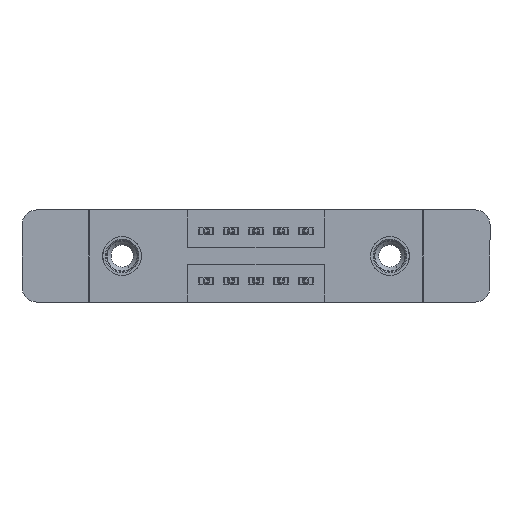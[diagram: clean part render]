
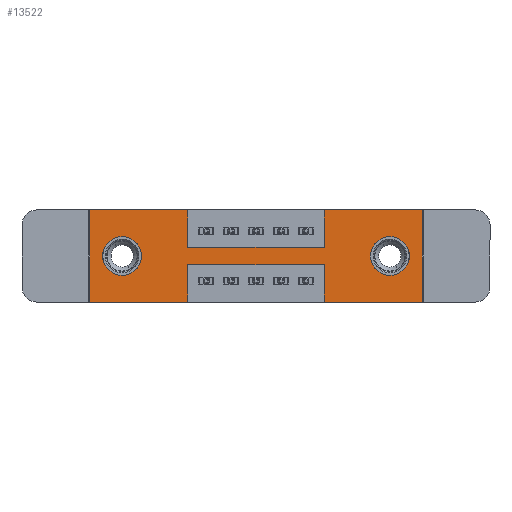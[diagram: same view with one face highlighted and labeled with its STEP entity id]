
A CAD part, front view. The second image highlights one B-rep face of the part: STEP entity #13522.
In plain terms, the highlighted planar face has unit normal (0, -1, 0).
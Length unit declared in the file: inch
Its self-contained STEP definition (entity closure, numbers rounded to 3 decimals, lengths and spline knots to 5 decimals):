
#14 = ORIENTED_EDGE ( 'NONE', *, *, #12716, .F. ) ;
#40 = CARTESIAN_POINT ( 'NONE',  ( 0.3925, 0., -0.15 ) ) ;
#54 = VERTEX_POINT ( 'NONE', #1777 ) ;
#109 = DIRECTION ( 'NONE',  ( 0., 0., 1. ) ) ;
#143 = CARTESIAN_POINT ( 'NONE',  ( 0.13, 0., -0.263 ) ) ;
#145 = CIRCLE ( 'NONE', #7231, 0.078 ) ;
#242 = CIRCLE ( 'NONE', #5730, 0.078 ) ;
#367 = DIRECTION ( 'NONE',  ( 0., 0., 1. ) ) ;
#396 = VERTEX_POINT ( 'NONE', #4580 ) ;
#408 = EDGE_CURVE ( 'NONE', #1911, #396, #1537, .T. ) ;
#434 = VECTOR ( 'NONE', #10616, 39.37008 ) ;
#489 = EDGE_CURVE ( 'NONE', #2141, #800, #8428, .T. ) ;
#511 = CARTESIAN_POINT ( 'NONE',  ( 0.9425, 0., 0. ) ) ;
#569 = DIRECTION ( 'NONE',  ( 0., 0., -1. ) ) ;
#647 = DIRECTION ( 'NONE',  ( -1., 0., 0. ) ) ;
#788 = CARTESIAN_POINT ( 'NONE',  ( 0.3925, 0., -0.37 ) ) ;
#800 = VERTEX_POINT ( 'NONE', #5962 ) ;
#908 = VERTEX_POINT ( 'NONE', #143 ) ;
#941 = ORIENTED_EDGE ( 'NONE', *, *, #489, .F. ) ;
#1104 = VERTEX_POINT ( 'NONE', #11388 ) ;
#1537 = CIRCLE ( 'NONE', #7495, 0.078 ) ;
#1569 = CARTESIAN_POINT ( 'NONE',  ( 0., 0., -0.37 ) ) ;
#1573 = CIRCLE ( 'NONE', #5460, 0.078 ) ;
#1625 = DIRECTION ( 'NONE',  ( 0., 1., 0. ) ) ;
#1772 = EDGE_CURVE ( 'NONE', #54, #3275, #6254, .T. ) ;
#1777 = CARTESIAN_POINT ( 'NONE',  ( 0.9425, 0., -0.22 ) ) ;
#1802 = CARTESIAN_POINT ( 'NONE',  ( 0.9425, 0., -0.37 ) ) ;
#1911 = VERTEX_POINT ( 'NONE', #5954 ) ;
#1930 = ORIENTED_EDGE ( 'NONE', *, *, #1772, .F. ) ;
#2028 = CARTESIAN_POINT ( 'NONE',  ( 0.9425, 0., -0.37 ) ) ;
#2094 = ORIENTED_EDGE ( 'NONE', *, *, #10803, .F. ) ;
#2141 = VERTEX_POINT ( 'NONE', #4910 ) ;
#2240 = CARTESIAN_POINT ( 'NONE',  ( 1.205, 0., -0.185 ) ) ;
#2312 = EDGE_CURVE ( 'NONE', #8408, #2580, #8908, .T. ) ;
#2437 = VERTEX_POINT ( 'NONE', #9054 ) ;
#2528 = VECTOR ( 'NONE', #7247, 39.37008 ) ;
#2580 = VERTEX_POINT ( 'NONE', #13516 ) ;
#2590 = DIRECTION ( 'NONE',  ( 0., -1., 0. ) ) ;
#2774 = CARTESIAN_POINT ( 'NONE',  ( 0., 0., -0.37 ) ) ;
#2799 = ORIENTED_EDGE ( 'NONE', *, *, #12905, .T. ) ;
#2869 = LINE ( 'NONE', #7093, #11901 ) ;
#2993 = DIRECTION ( 'NONE',  ( 0., 0., -1. ) ) ;
#3033 = EDGE_CURVE ( 'NONE', #3275, #1104, #11607, .T. ) ;
#3177 = LINE ( 'NONE', #13793, #10722 ) ;
#3210 = DIRECTION ( 'NONE',  ( 0., 0., 1. ) ) ;
#3251 = ORIENTED_EDGE ( 'NONE', *, *, #6600, .F. ) ;
#3275 = VERTEX_POINT ( 'NONE', #3446 ) ;
#3441 = CARTESIAN_POINT ( 'NONE',  ( 0.9425, 0., 0. ) ) ;
#3446 = CARTESIAN_POINT ( 'NONE',  ( 0.3925, 0., -0.22 ) ) ;
#3498 = DIRECTION ( 'NONE',  ( 0., 1., 0. ) ) ;
#3857 = VECTOR ( 'NONE', #13791, 39.37008 ) ;
#3929 = CARTESIAN_POINT ( 'NONE',  ( 1.335, 0., 0. ) ) ;
#3960 = ORIENTED_EDGE ( 'NONE', *, *, #13462, .F. ) ;
#4412 = DIRECTION ( 'NONE',  ( 1., 0., 0. ) ) ;
#4465 = DIRECTION ( 'NONE',  ( 0., 0., -1. ) ) ;
#4484 = DIRECTION ( 'NONE',  ( 0., 0., 1. ) ) ;
#4497 = VECTOR ( 'NONE', #4484, 39.37008 ) ;
#4580 = CARTESIAN_POINT ( 'NONE',  ( 1.205, 0., -0.263 ) ) ;
#4705 = VECTOR ( 'NONE', #2993, 39.37008 ) ;
#4761 = EDGE_LOOP ( 'NONE', ( #12959, #2799 ) ) ;
#4842 = ORIENTED_EDGE ( 'NONE', *, *, #13003, .F. ) ;
#4910 = CARTESIAN_POINT ( 'NONE',  ( 1.335, 0., 0. ) ) ;
#5101 = ORIENTED_EDGE ( 'NONE', *, *, #8015, .F. ) ;
#5460 = AXIS2_PLACEMENT_3D ( 'NONE', #2240, #13506, #4465 ) ;
#5730 = AXIS2_PLACEMENT_3D ( 'NONE', #5948, #12604, #109 ) ;
#5835 = ORIENTED_EDGE ( 'NONE', *, *, #12366, .F. ) ;
#5948 = CARTESIAN_POINT ( 'NONE',  ( 0.13, 0., -0.185 ) ) ;
#5954 = CARTESIAN_POINT ( 'NONE',  ( 1.205, 0., -0.107 ) ) ;
#5962 = CARTESIAN_POINT ( 'NONE',  ( 1.335, 0., -0.37 ) ) ;
#6108 = VECTOR ( 'NONE', #13656, 39.37008 ) ;
#6136 = LINE ( 'NONE', #11443, #4705 ) ;
#6254 = LINE ( 'NONE', #14079, #434 ) ;
#6389 = VECTOR ( 'NONE', #367, 39.37008 ) ;
#6572 = VERTEX_POINT ( 'NONE', #10578 ) ;
#6600 = EDGE_CURVE ( 'NONE', #2437, #8408, #6136, .T. ) ;
#7039 = VECTOR ( 'NONE', #7356, 39.37008 ) ;
#7068 = LINE ( 'NONE', #2774, #6108 ) ;
#7093 = CARTESIAN_POINT ( 'NONE',  ( 0., 0., -0.37 ) ) ;
#7224 = VERTEX_POINT ( 'NONE', #2028 ) ;
#7231 = AXIS2_PLACEMENT_3D ( 'NONE', #11948, #3498, #3210 ) ;
#7247 = DIRECTION ( 'NONE',  ( 0., 0., 1. ) ) ;
#7282 = CARTESIAN_POINT ( 'NONE',  ( 1.205, 0., -0.185 ) ) ;
#7356 = DIRECTION ( 'NONE',  ( 0., 0., -1. ) ) ;
#7495 = AXIS2_PLACEMENT_3D ( 'NONE', #7282, #1625, #11649 ) ;
#8015 = EDGE_CURVE ( 'NONE', #9460, #6572, #8506, .T. ) ;
#8163 = PLANE ( 'NONE',  #10294 ) ;
#8310 = EDGE_LOOP ( 'NONE', ( #13351, #1930, #4842, #3960, #941, #8535, #14, #8772, #3251, #5835, #5101, #2094 ) ) ;
#8333 = VERTEX_POINT ( 'NONE', #9343 ) ;
#8399 = CARTESIAN_POINT ( 'NONE',  ( 0., 0., 0. ) ) ;
#8408 = VERTEX_POINT ( 'NONE', #10776 ) ;
#8428 = LINE ( 'NONE', #3929, #7039 ) ;
#8506 = LINE ( 'NONE', #8836, #4497 ) ;
#8535 = ORIENTED_EDGE ( 'NONE', *, *, #11397, .F. ) ;
#8772 = ORIENTED_EDGE ( 'NONE', *, *, #2312, .F. ) ;
#8836 = CARTESIAN_POINT ( 'NONE',  ( 0., 0., 0. ) ) ;
#8908 = LINE ( 'NONE', #40, #12082 ) ;
#9054 = CARTESIAN_POINT ( 'NONE',  ( 0.3925, 0., 0. ) ) ;
#9343 = CARTESIAN_POINT ( 'NONE',  ( 0.13, 0., -0.107 ) ) ;
#9457 = EDGE_CURVE ( 'NONE', #8333, #908, #145, .T. ) ;
#9460 = VERTEX_POINT ( 'NONE', #13091 ) ;
#9608 = VECTOR ( 'NONE', #12965, 39.37008 ) ;
#9857 = EDGE_LOOP ( 'NONE', ( #10556, #12037 ) ) ;
#10169 = FACE_BOUND ( 'NONE', #4761, .T. ) ;
#10198 = VERTEX_POINT ( 'NONE', #3441 ) ;
#10243 = FACE_OUTER_BOUND ( 'NONE', #8310, .T. ) ;
#10294 = AXIS2_PLACEMENT_3D ( 'NONE', #1569, #2590, #569 ) ;
#10556 = ORIENTED_EDGE ( 'NONE', *, *, #9457, .T. ) ;
#10578 = CARTESIAN_POINT ( 'NONE',  ( 0., 0., 0. ) ) ;
#10616 = DIRECTION ( 'NONE',  ( -1., 0., 0. ) ) ;
#10722 = VECTOR ( 'NONE', #14015, 39.37008 ) ;
#10776 = CARTESIAN_POINT ( 'NONE',  ( 0.3925, 0., -0.15 ) ) ;
#10803 = EDGE_CURVE ( 'NONE', #1104, #9460, #7068, .T. ) ;
#11388 = CARTESIAN_POINT ( 'NONE',  ( 0.3925, 0., -0.37 ) ) ;
#11397 = EDGE_CURVE ( 'NONE', #10198, #2141, #12692, .T. ) ;
#11443 = CARTESIAN_POINT ( 'NONE',  ( 0.3925, 0., 0. ) ) ;
#11607 = LINE ( 'NONE', #788, #9608 ) ;
#11649 = DIRECTION ( 'NONE',  ( 0., 0., -1. ) ) ;
#11901 = VECTOR ( 'NONE', #647, 39.37008 ) ;
#11948 = CARTESIAN_POINT ( 'NONE',  ( 0.13, 0., -0.185 ) ) ;
#12037 = ORIENTED_EDGE ( 'NONE', *, *, #13544, .T. ) ;
#12082 = VECTOR ( 'NONE', #4412, 39.37008 ) ;
#12366 = EDGE_CURVE ( 'NONE', #6572, #2437, #3177, .T. ) ;
#12460 = FACE_BOUND ( 'NONE', #9857, .T. ) ;
#12604 = DIRECTION ( 'NONE',  ( 0., 1., 0. ) ) ;
#12692 = LINE ( 'NONE', #8399, #3857 ) ;
#12716 = EDGE_CURVE ( 'NONE', #2580, #10198, #13421, .T. ) ;
#12905 = EDGE_CURVE ( 'NONE', #396, #1911, #1573, .T. ) ;
#12959 = ORIENTED_EDGE ( 'NONE', *, *, #408, .T. ) ;
#12965 = DIRECTION ( 'NONE',  ( 0., 0., -1. ) ) ;
#13003 = EDGE_CURVE ( 'NONE', #7224, #54, #13631, .T. ) ;
#13091 = CARTESIAN_POINT ( 'NONE',  ( 0., 0., -0.37 ) ) ;
#13351 = ORIENTED_EDGE ( 'NONE', *, *, #3033, .F. ) ;
#13421 = LINE ( 'NONE', #511, #6389 ) ;
#13462 = EDGE_CURVE ( 'NONE', #800, #7224, #2869, .T. ) ;
#13506 = DIRECTION ( 'NONE',  ( 0., 1., 0. ) ) ;
#13516 = CARTESIAN_POINT ( 'NONE',  ( 0.9425, 0., -0.15 ) ) ;
#13522 = ADVANCED_FACE ( 'NONE', ( #10169, #12460, #10243 ), #8163, .T. ) ;
#13544 = EDGE_CURVE ( 'NONE', #908, #8333, #242, .T. ) ;
#13631 = LINE ( 'NONE', #1802, #2528 ) ;
#13656 = DIRECTION ( 'NONE',  ( -1., 0., 0. ) ) ;
#13791 = DIRECTION ( 'NONE',  ( 1., 0., 0. ) ) ;
#13793 = CARTESIAN_POINT ( 'NONE',  ( 0., 0., 0. ) ) ;
#14015 = DIRECTION ( 'NONE',  ( 1., 0., 0. ) ) ;
#14079 = CARTESIAN_POINT ( 'NONE',  ( 0.3925, 0., -0.22 ) ) ;
